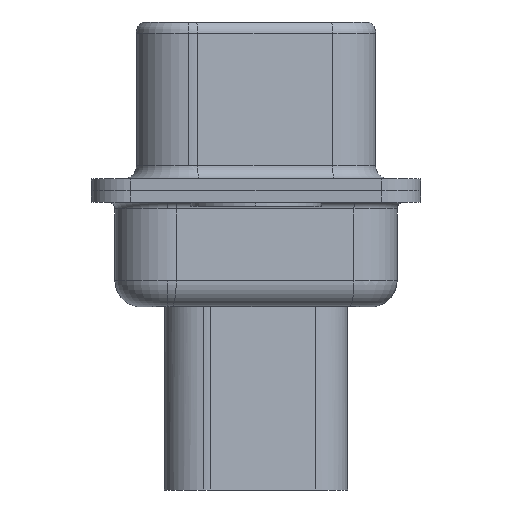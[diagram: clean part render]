
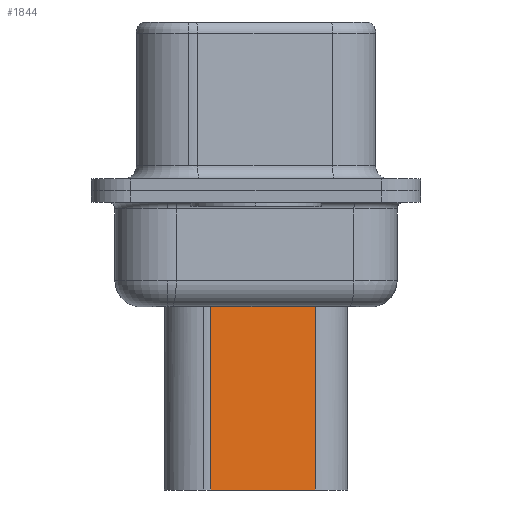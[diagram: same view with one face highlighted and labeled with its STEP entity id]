
A CAD part, left-side view. The second image highlights one B-rep face of the part: STEP entity #1844.
In plain terms, the highlighted planar face has unit normal (-0.985, -0.174, 0).
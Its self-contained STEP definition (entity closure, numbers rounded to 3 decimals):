
#553 = CARTESIAN_POINT ( 'NONE',  ( 4.524, 1.74, -11.45 ) ) ;
#706 = FACE_OUTER_BOUND ( 'NONE', #13386, .T. ) ;
#1844 = ADVANCED_FACE ( 'NONE', ( #706 ), #10198, .T. ) ;
#2018 = VECTOR ( 'NONE', #3830, 1000. ) ;
#2780 = VECTOR ( 'NONE', #13238, 1000. ) ;
#3161 = CARTESIAN_POINT ( 'NONE',  ( 4.524, 1.74, -3.975 ) ) ;
#3177 = LINE ( 'NONE', #553, #2780 ) ;
#3493 = DIRECTION ( 'NONE',  ( 0., 0., -1. ) ) ;
#3830 = DIRECTION ( 'NONE',  ( 0., 0., -1. ) ) ;
#3874 = AXIS2_PLACEMENT_3D ( 'NONE', #11758, #8801, #16060 ) ;
#3917 = CARTESIAN_POINT ( 'NONE',  ( 5.229, -2.26, -11.45 ) ) ;
#5354 = LINE ( 'NONE', #11424, #2018 ) ;
#5625 = EDGE_CURVE ( 'NONE', #15622, #8690, #16321, .T. ) ;
#5670 = VERTEX_POINT ( 'NONE', #3917 ) ;
#6251 = CARTESIAN_POINT ( 'NONE',  ( 4.524, 1.74, -11.45 ) ) ;
#7249 = ORIENTED_EDGE ( 'NONE', *, *, #14383, .F. ) ;
#8690 = VERTEX_POINT ( 'NONE', #3161 ) ;
#8737 = VECTOR ( 'NONE', #3493, 1000. ) ;
#8783 = EDGE_CURVE ( 'NONE', #8690, #11271, #12132, .T. ) ;
#8801 = DIRECTION ( 'NONE',  ( -0.985, -0.174, 0. ) ) ;
#8855 = DIRECTION ( 'NONE',  ( -0.174, 0.985, 0. ) ) ;
#9480 = ORIENTED_EDGE ( 'NONE', *, *, #5625, .T. ) ;
#10188 = CARTESIAN_POINT ( 'NONE',  ( 4.353, 2.709, -3.975 ) ) ;
#10198 = PLANE ( 'NONE',  #3874 ) ;
#11271 = VERTEX_POINT ( 'NONE', #6251 ) ;
#11381 = ORIENTED_EDGE ( 'NONE', *, *, #8783, .T. ) ;
#11424 = CARTESIAN_POINT ( 'NONE',  ( 5.229, -2.26, -3.1 ) ) ;
#11758 = CARTESIAN_POINT ( 'NONE',  ( 4.524, 1.74, -3.1 ) ) ;
#11934 = EDGE_CURVE ( 'NONE', #15622, #5670, #5354, .T. ) ;
#12132 = LINE ( 'NONE', #16114, #8737 ) ;
#12173 = VECTOR ( 'NONE', #8855, 1000. ) ;
#13238 = DIRECTION ( 'NONE',  ( -0.174, 0.985, 0. ) ) ;
#13386 = EDGE_LOOP ( 'NONE', ( #15997, #9480, #11381, #7249 ) ) ;
#14383 = EDGE_CURVE ( 'NONE', #5670, #11271, #3177, .T. ) ;
#15138 = CARTESIAN_POINT ( 'NONE',  ( 5.229, -2.26, -3.975 ) ) ;
#15622 = VERTEX_POINT ( 'NONE', #15138 ) ;
#15997 = ORIENTED_EDGE ( 'NONE', *, *, #11934, .F. ) ;
#16060 = DIRECTION ( 'NONE',  ( 0.174, -0.985, 0. ) ) ;
#16114 = CARTESIAN_POINT ( 'NONE',  ( 4.524, 1.74, -3.1 ) ) ;
#16321 = LINE ( 'NONE', #10188, #12173 ) ;
